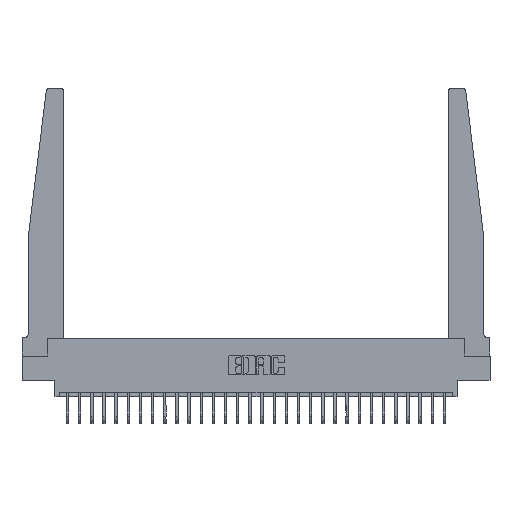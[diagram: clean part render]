
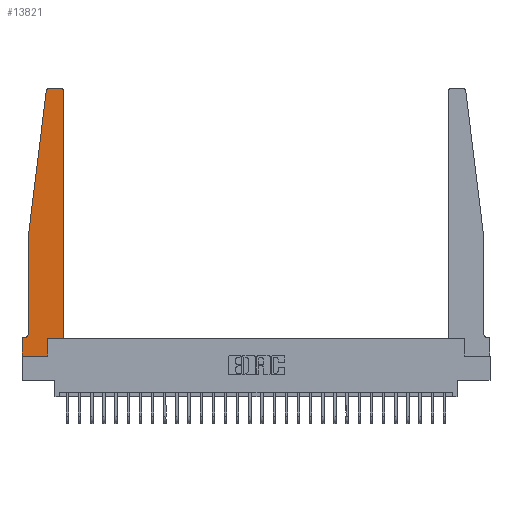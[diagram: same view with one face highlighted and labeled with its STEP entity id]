
A CAD part, top view. The second image highlights one B-rep face of the part: STEP entity #13821.
In plain terms, the highlighted planar face has unit normal (0, 0, 1).
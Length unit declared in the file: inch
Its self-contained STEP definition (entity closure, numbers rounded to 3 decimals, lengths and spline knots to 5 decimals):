
#250 = CARTESIAN_POINT ( 'NONE',  ( 0.27653, 2.75, 0.37 ) ) ;
#630 = VECTOR ( 'NONE', #6205, 39.37008 ) ;
#725 = EDGE_CURVE ( 'NONE', #3619, #23081, #19514, .T. ) ;
#1190 = PLANE ( 'NONE',  #27146 ) ;
#1515 = CARTESIAN_POINT ( 'NONE',  ( 0.24675, 2.72367, 0.37 ) ) ;
#1569 = CARTESIAN_POINT ( 'NONE',  ( 0., 0., 0.37 ) ) ;
#1797 = CIRCLE ( 'NONE', #27890, 0.03 ) ;
#1890 = EDGE_CURVE ( 'NONE', #16605, #8330, #7979, .T. ) ;
#2545 = ORIENTED_EDGE ( 'NONE', *, *, #725, .T. ) ;
#2797 = VECTOR ( 'NONE', #15152, 39.37008 ) ;
#3155 = EDGE_CURVE ( 'NONE', #23081, #16605, #23205, .T. ) ;
#3273 = CARTESIAN_POINT ( 'NONE',  ( 0.015, 0.1875, 0.37 ) ) ;
#3307 = LINE ( 'NONE', #20351, #27364 ) ;
#3619 = VERTEX_POINT ( 'NONE', #20195 ) ;
#4260 = VERTEX_POINT ( 'NONE', #10869 ) ;
#5230 = ORIENTED_EDGE ( 'NONE', *, *, #12277, .T. ) ;
#5281 = VERTEX_POINT ( 'NONE', #19049 ) ;
#5757 = CARTESIAN_POINT ( 'NONE',  ( 0.25, 2.75, 0.37 ) ) ;
#5771 = VECTOR ( 'NONE', #16680, 39.37008 ) ;
#5833 = CARTESIAN_POINT ( 'NONE',  ( 0.395, 2.75, 0.37 ) ) ;
#6205 = DIRECTION ( 'NONE',  ( 0., -1., 0. ) ) ;
#6395 = CARTESIAN_POINT ( 'NONE',  ( 0., 0., 0.37 ) ) ;
#6658 = ORIENTED_EDGE ( 'NONE', *, *, #1890, .T. ) ;
#6901 = ORIENTED_EDGE ( 'NONE', *, *, #27412, .T. ) ;
#7009 = VECTOR ( 'NONE', #14632, 39.37008 ) ;
#7360 = CARTESIAN_POINT ( 'NONE',  ( 0.2605, 0.18, 0.37 ) ) ;
#7431 = VECTOR ( 'NONE', #11320, 39.37008 ) ;
#7979 = LINE ( 'NONE', #6395, #630 ) ;
#8178 = CARTESIAN_POINT ( 'NONE',  ( 0.065, 0.1875, 0.37 ) ) ;
#8285 = CARTESIAN_POINT ( 'NONE',  ( 0.2605, 0.18, 0.37 ) ) ;
#8330 = VERTEX_POINT ( 'NONE', #1569 ) ;
#8446 = CARTESIAN_POINT ( 'NONE',  ( 0.425, 0.18, 0.37 ) ) ;
#8833 = EDGE_CURVE ( 'NONE', #22549, #26924, #21280, .T. ) ;
#8893 = DIRECTION ( 'NONE',  ( 0., 0., 1. ) ) ;
#9648 = ORIENTED_EDGE ( 'NONE', *, *, #3155, .T. ) ;
#9701 = VERTEX_POINT ( 'NONE', #24475 ) ;
#9717 = LINE ( 'NONE', #12702, #2797 ) ;
#9816 = ORIENTED_EDGE ( 'NONE', *, *, #17781, .T. ) ;
#9974 = CARTESIAN_POINT ( 'NONE',  ( 0.015, 0.2375, 0.37 ) ) ;
#10643 = CARTESIAN_POINT ( 'NONE',  ( 0.425, 0.18, 0.37 ) ) ;
#10770 = VECTOR ( 'NONE', #18778, 39.37008 ) ;
#10869 = CARTESIAN_POINT ( 'NONE',  ( 0.2605, 0., 0.37 ) ) ;
#11046 = EDGE_CURVE ( 'NONE', #5281, #22549, #1797, .T. ) ;
#11320 = DIRECTION ( 'NONE',  ( 1., 0., 0. ) ) ;
#11995 = VERTEX_POINT ( 'NONE', #8285 ) ;
#12134 = AXIS2_PLACEMENT_3D ( 'NONE', #9974, #23094, #20929 ) ;
#12277 = EDGE_CURVE ( 'NONE', #11995, #9701, #16408, .T. ) ;
#12702 = CARTESIAN_POINT ( 'NONE',  ( 0.065, 1.25, 0.37 ) ) ;
#12793 = EDGE_CURVE ( 'NONE', #26924, #25500, #25144, .T. ) ;
#13125 = ORIENTED_EDGE ( 'NONE', *, *, #25179, .T. ) ;
#13145 = EDGE_LOOP ( 'NONE', ( #25704, #15105, #19307, #6901, #2545, #9648, #6658, #13125, #9816, #5230, #19545, #28720 ) ) ;
#13338 = CARTESIAN_POINT ( 'NONE',  ( 0.395, 2.72, 0.37 ) ) ;
#13821 = ADVANCED_FACE ( 'NONE', ( #28593 ), #1190, .T. ) ;
#14184 = VERTEX_POINT ( 'NONE', #22460 ) ;
#14583 = CARTESIAN_POINT ( 'NONE',  ( 0., 0.1875, 0.37 ) ) ;
#14632 = DIRECTION ( 'NONE',  ( 0., 1., 0. ) ) ;
#15105 = ORIENTED_EDGE ( 'NONE', *, *, #12793, .T. ) ;
#15152 = DIRECTION ( 'NONE',  ( 0., -1., 0. ) ) ;
#15702 = VECTOR ( 'NONE', #17389, 39.37008 ) ;
#15912 = CARTESIAN_POINT ( 'NONE',  ( 0., 0., 0.37 ) ) ;
#16307 = EDGE_CURVE ( 'NONE', #25500, #14184, #3307, .T. ) ;
#16408 = LINE ( 'NONE', #10643, #15702 ) ;
#16605 = VERTEX_POINT ( 'NONE', #19252 ) ;
#16680 = DIRECTION ( 'NONE',  ( -1., 0., 0. ) ) ;
#17389 = DIRECTION ( 'NONE',  ( 1., 0., 0. ) ) ;
#17433 = CARTESIAN_POINT ( 'NONE',  ( 0.27653, 2.72, 0.37 ) ) ;
#17781 = EDGE_CURVE ( 'NONE', #4260, #11995, #20283, .T. ) ;
#18778 = DIRECTION ( 'NONE',  ( 0., 1., 0. ) ) ;
#19049 = CARTESIAN_POINT ( 'NONE',  ( 0.425, 2.72, 0.37 ) ) ;
#19203 = DIRECTION ( 'NONE',  ( -1., 0., 0. ) ) ;
#19219 = DIRECTION ( 'NONE',  ( 1., 0., 0. ) ) ;
#19252 = CARTESIAN_POINT ( 'NONE',  ( 0., 0.1875, 0.37 ) ) ;
#19307 = ORIENTED_EDGE ( 'NONE', *, *, #16307, .T. ) ;
#19514 = CIRCLE ( 'NONE', #12134, 0.05 ) ;
#19545 = ORIENTED_EDGE ( 'NONE', *, *, #20365, .T. ) ;
#19688 = LINE ( 'NONE', #15912, #7431 ) ;
#19721 = DIRECTION ( 'NONE',  ( 0., 0., 1. ) ) ;
#19901 = VECTOR ( 'NONE', #19203, 39.37008 ) ;
#20195 = CARTESIAN_POINT ( 'NONE',  ( 0.065, 0.2375, 0.37 ) ) ;
#20283 = LINE ( 'NONE', #7360, #10770 ) ;
#20351 = CARTESIAN_POINT ( 'NONE',  ( 0.065, 1.25, 0.37 ) ) ;
#20365 = EDGE_CURVE ( 'NONE', #9701, #5281, #27241, .T. ) ;
#20929 = DIRECTION ( 'NONE',  ( -1., 0., 0. ) ) ;
#21273 = DIRECTION ( 'NONE',  ( 0., 0., 1. ) ) ;
#21280 = LINE ( 'NONE', #5757, #19901 ) ;
#22277 = AXIS2_PLACEMENT_3D ( 'NONE', #17433, #19721, #26437 ) ;
#22460 = CARTESIAN_POINT ( 'NONE',  ( 0.065, 1.25, 0.37 ) ) ;
#22549 = VERTEX_POINT ( 'NONE', #5833 ) ;
#23081 = VERTEX_POINT ( 'NONE', #3273 ) ;
#23094 = DIRECTION ( 'NONE',  ( 0., 0., -1. ) ) ;
#23205 = LINE ( 'NONE', #8178, #5771 ) ;
#24475 = CARTESIAN_POINT ( 'NONE',  ( 0.425, 0.18, 0.37 ) ) ;
#24648 = DIRECTION ( 'NONE',  ( -0.122, -0.992, 0. ) ) ;
#25144 = CIRCLE ( 'NONE', #22277, 0.03 ) ;
#25179 = EDGE_CURVE ( 'NONE', #8330, #4260, #19688, .T. ) ;
#25500 = VERTEX_POINT ( 'NONE', #1515 ) ;
#25704 = ORIENTED_EDGE ( 'NONE', *, *, #8833, .T. ) ;
#26437 = DIRECTION ( 'NONE',  ( 1., 0., 0. ) ) ;
#26924 = VERTEX_POINT ( 'NONE', #250 ) ;
#27146 = AXIS2_PLACEMENT_3D ( 'NONE', #14583, #21273, #19219 ) ;
#27241 = LINE ( 'NONE', #8446, #7009 ) ;
#27364 = VECTOR ( 'NONE', #24648, 39.37008 ) ;
#27412 = EDGE_CURVE ( 'NONE', #14184, #3619, #9717, .T. ) ;
#27890 = AXIS2_PLACEMENT_3D ( 'NONE', #13338, #8893, #28814 ) ;
#28593 = FACE_OUTER_BOUND ( 'NONE', #13145, .T. ) ;
#28720 = ORIENTED_EDGE ( 'NONE', *, *, #11046, .T. ) ;
#28814 = DIRECTION ( 'NONE',  ( 1., 0., 0. ) ) ;
